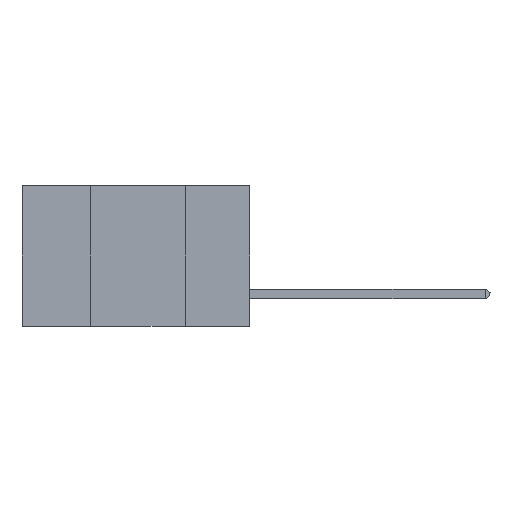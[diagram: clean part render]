
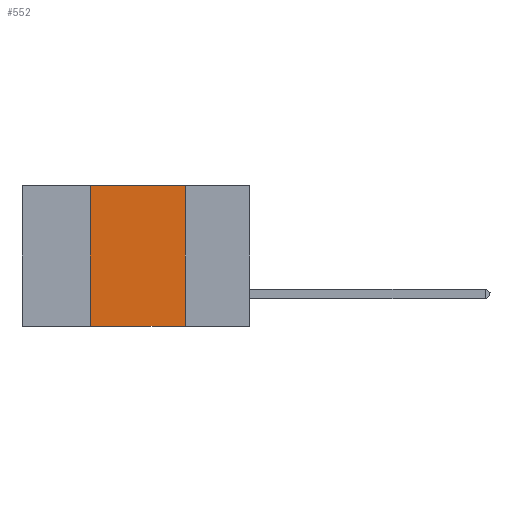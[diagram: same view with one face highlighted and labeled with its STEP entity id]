
A CAD part, left-side view. The second image highlights one B-rep face of the part: STEP entity #552.
In plain terms, the highlighted planar face has unit normal (-1, 0, 0).
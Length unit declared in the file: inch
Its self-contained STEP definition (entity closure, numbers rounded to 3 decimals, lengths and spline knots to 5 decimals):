
#255 = VECTOR ( 'NONE', #4852, 39.37008 ) ;
#280 = LINE ( 'NONE', #13112, #1242 ) ;
#552 = ADVANCED_FACE ( 'NONE', ( #4983 ), #1592, .F. ) ;
#1242 = VECTOR ( 'NONE', #10221, 39.37008 ) ;
#1265 = ORIENTED_EDGE ( 'NONE', *, *, #8177, .T. ) ;
#1592 = PLANE ( 'NONE',  #12525 ) ;
#1681 = CARTESIAN_POINT ( 'NONE',  ( 0., 0.42, -0.37 ) ) ;
#2503 = VERTEX_POINT ( 'NONE', #3802 ) ;
#2874 = VECTOR ( 'NONE', #4706, 39.37008 ) ;
#3417 = EDGE_CURVE ( 'NONE', #2503, #11594, #280, .T. ) ;
#3802 = CARTESIAN_POINT ( 'NONE',  ( 0., 0.17, 0. ) ) ;
#4579 = ORIENTED_EDGE ( 'NONE', *, *, #10340, .F. ) ;
#4614 = LINE ( 'NONE', #6597, #2874 ) ;
#4706 = DIRECTION ( 'NONE',  ( 0., -1., 0. ) ) ;
#4852 = DIRECTION ( 'NONE',  ( 0., 0., 1. ) ) ;
#4983 = FACE_OUTER_BOUND ( 'NONE', #9685, .T. ) ;
#5735 = VERTEX_POINT ( 'NONE', #1681 ) ;
#6032 = LINE ( 'NONE', #8225, #7313 ) ;
#6343 = DIRECTION ( 'NONE',  ( 0., -1., 0. ) ) ;
#6597 = CARTESIAN_POINT ( 'NONE',  ( 0., 0.6, -0.37 ) ) ;
#7007 = ORIENTED_EDGE ( 'NONE', *, *, #9232, .F. ) ;
#7313 = VECTOR ( 'NONE', #6343, 39.37008 ) ;
#7662 = CARTESIAN_POINT ( 'NONE',  ( 0., 0.6, 0. ) ) ;
#7726 = CARTESIAN_POINT ( 'NONE',  ( 0., 0.42, 0. ) ) ;
#8177 = EDGE_CURVE ( 'NONE', #5735, #11594, #4614, .T. ) ;
#8216 = VERTEX_POINT ( 'NONE', #7726 ) ;
#8225 = CARTESIAN_POINT ( 'NONE',  ( 0., 0.6, 0. ) ) ;
#9197 = LINE ( 'NONE', #11282, #255 ) ;
#9232 = EDGE_CURVE ( 'NONE', #8216, #2503, #6032, .T. ) ;
#9356 = ORIENTED_EDGE ( 'NONE', *, *, #3417, .F. ) ;
#9685 = EDGE_LOOP ( 'NONE', ( #9356, #7007, #4579, #1265 ) ) ;
#9855 = CARTESIAN_POINT ( 'NONE',  ( 0., 0.17, -0.37 ) ) ;
#10221 = DIRECTION ( 'NONE',  ( 0., 0., -1. ) ) ;
#10340 = EDGE_CURVE ( 'NONE', #5735, #8216, #9197, .T. ) ;
#10561 = DIRECTION ( 'NONE',  ( 0., 0., -1. ) ) ;
#11282 = CARTESIAN_POINT ( 'NONE',  ( 0., 0.42, 0. ) ) ;
#11594 = VERTEX_POINT ( 'NONE', #9855 ) ;
#12525 = AXIS2_PLACEMENT_3D ( 'NONE', #7662, #12605, #10561 ) ;
#12605 = DIRECTION ( 'NONE',  ( 1., 0., 0. ) ) ;
#13112 = CARTESIAN_POINT ( 'NONE',  ( 0., 0.17, 0. ) ) ;
